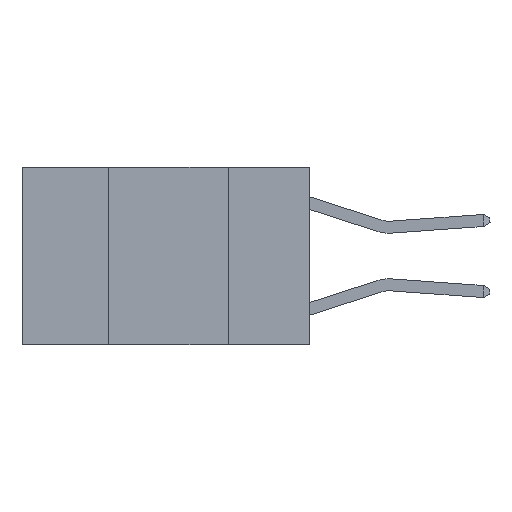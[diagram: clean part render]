
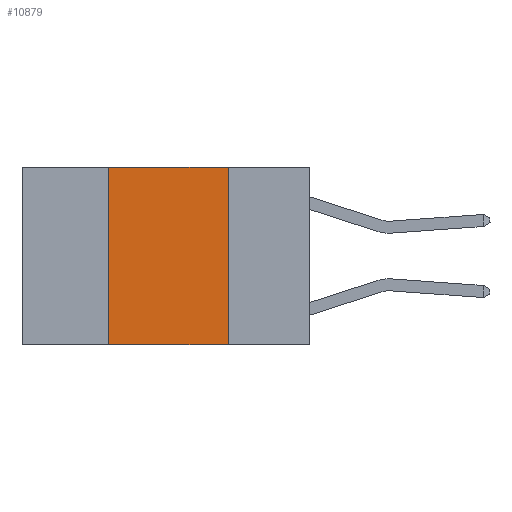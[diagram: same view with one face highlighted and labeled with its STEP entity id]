
A CAD part, left-side view. The second image highlights one B-rep face of the part: STEP entity #10879.
In plain terms, the highlighted planar face has unit normal (-1, 0, 0).
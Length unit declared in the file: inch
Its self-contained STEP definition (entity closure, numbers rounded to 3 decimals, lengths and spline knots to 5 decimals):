
#207 = LINE ( 'NONE', #9611, #2437 ) ;
#813 = VECTOR ( 'NONE', #4924, 39.37008 ) ;
#1375 = CARTESIAN_POINT ( 'NONE',  ( 0., 0.6, -0.37 ) ) ;
#1677 = CARTESIAN_POINT ( 'NONE',  ( 0., 0.6, 0. ) ) ;
#2437 = VECTOR ( 'NONE', #2768, 39.37008 ) ;
#2476 = EDGE_CURVE ( 'NONE', #5360, #3255, #7874, .T. ) ;
#2490 = EDGE_CURVE ( 'NONE', #5360, #6947, #9235, .T. ) ;
#2492 = EDGE_CURVE ( 'NONE', #8479, #6947, #207, .T. ) ;
#2615 = DIRECTION ( 'NONE',  ( 0., 0., -1. ) ) ;
#2736 = VECTOR ( 'NONE', #3225, 39.37008 ) ;
#2748 = EDGE_CURVE ( 'NONE', #3255, #8479, #6030, .T. ) ;
#2768 = DIRECTION ( 'NONE',  ( 0., 0., -1. ) ) ;
#2876 = ORIENTED_EDGE ( 'NONE', *, *, #2748, .F. ) ;
#2952 = CARTESIAN_POINT ( 'NONE',  ( 0., 0.42, -0.37 ) ) ;
#3225 = DIRECTION ( 'NONE',  ( 0., -1., 0. ) ) ;
#3255 = VERTEX_POINT ( 'NONE', #6209 ) ;
#4032 = AXIS2_PLACEMENT_3D ( 'NONE', #1677, #7809, #2615 ) ;
#4579 = EDGE_LOOP ( 'NONE', ( #10531, #2876, #8024, #8475 ) ) ;
#4924 = DIRECTION ( 'NONE',  ( 0., 0., 1. ) ) ;
#5360 = VERTEX_POINT ( 'NONE', #2952 ) ;
#6030 = LINE ( 'NONE', #9173, #9965 ) ;
#6074 = FACE_OUTER_BOUND ( 'NONE', #4579, .T. ) ;
#6209 = CARTESIAN_POINT ( 'NONE',  ( 0., 0.42, 0. ) ) ;
#6848 = CARTESIAN_POINT ( 'NONE',  ( 0., 0.42, 0. ) ) ;
#6947 = VERTEX_POINT ( 'NONE', #9011 ) ;
#7809 = DIRECTION ( 'NONE',  ( 1., 0., 0. ) ) ;
#7874 = LINE ( 'NONE', #6848, #813 ) ;
#8024 = ORIENTED_EDGE ( 'NONE', *, *, #2476, .F. ) ;
#8475 = ORIENTED_EDGE ( 'NONE', *, *, #2490, .T. ) ;
#8479 = VERTEX_POINT ( 'NONE', #9328 ) ;
#9011 = CARTESIAN_POINT ( 'NONE',  ( 0., 0.17, -0.37 ) ) ;
#9173 = CARTESIAN_POINT ( 'NONE',  ( 0., 0.6, 0. ) ) ;
#9235 = LINE ( 'NONE', #1375, #2736 ) ;
#9328 = CARTESIAN_POINT ( 'NONE',  ( 0., 0.17, 0. ) ) ;
#9369 = PLANE ( 'NONE',  #4032 ) ;
#9611 = CARTESIAN_POINT ( 'NONE',  ( 0., 0.17, 0. ) ) ;
#9960 = DIRECTION ( 'NONE',  ( 0., -1., 0. ) ) ;
#9965 = VECTOR ( 'NONE', #9960, 39.37008 ) ;
#10531 = ORIENTED_EDGE ( 'NONE', *, *, #2492, .F. ) ;
#10879 = ADVANCED_FACE ( 'NONE', ( #6074 ), #9369, .F. ) ;
